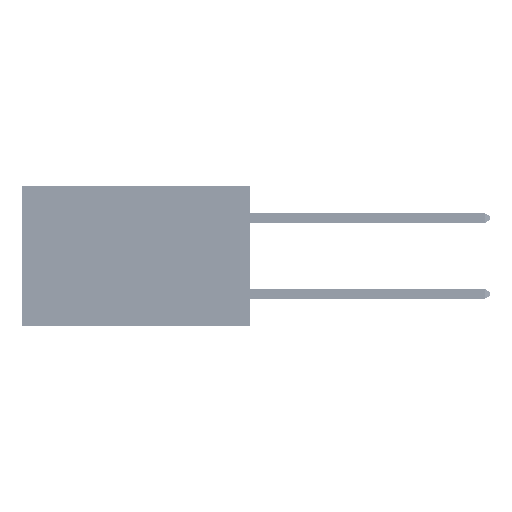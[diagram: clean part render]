
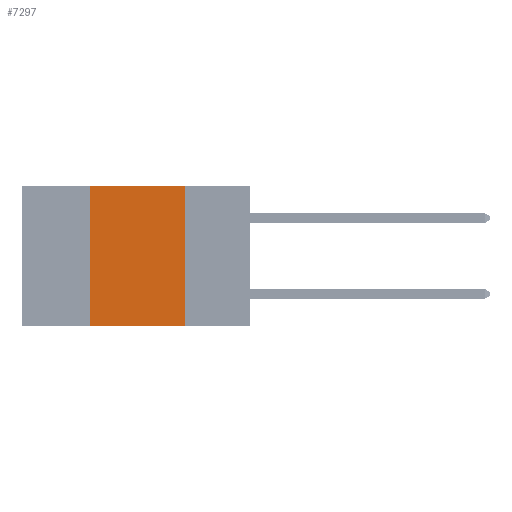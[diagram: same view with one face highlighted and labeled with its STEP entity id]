
A CAD part, left-side view. The second image highlights one B-rep face of the part: STEP entity #7297.
In plain terms, the highlighted planar face has unit normal (-1, 0, 0).
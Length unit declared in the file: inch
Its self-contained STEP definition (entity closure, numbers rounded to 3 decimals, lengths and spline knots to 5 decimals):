
#2633 = VERTEX_POINT ( 'NONE', #10321 ) ;
#2894 = ORIENTED_EDGE ( 'NONE', *, *, #41545, .F. ) ;
#4387 = CARTESIAN_POINT ( 'NONE',  ( 0., 0.17, 0. ) ) ;
#5004 = VECTOR ( 'NONE', #29606, 39.37008 ) ;
#6440 = ORIENTED_EDGE ( 'NONE', *, *, #28216, .T. ) ;
#6649 = CARTESIAN_POINT ( 'NONE',  ( 0., 0.42, 0. ) ) ;
#7297 = ADVANCED_FACE ( 'NONE', ( #26547 ), #14944, .F. ) ;
#7393 = CARTESIAN_POINT ( 'NONE',  ( 0., 0.6, 0. ) ) ;
#8429 = DIRECTION ( 'NONE',  ( 0., 0., -1. ) ) ;
#8774 = LINE ( 'NONE', #33139, #5004 ) ;
#9118 = DIRECTION ( 'NONE',  ( 0., 0., -1. ) ) ;
#10321 = CARTESIAN_POINT ( 'NONE',  ( 0., 0.17, -0.37 ) ) ;
#12246 = CARTESIAN_POINT ( 'NONE',  ( 0., 0.6, 0. ) ) ;
#13129 = VERTEX_POINT ( 'NONE', #13296 ) ;
#13296 = CARTESIAN_POINT ( 'NONE',  ( 0., 0.42, -0.37 ) ) ;
#14944 = PLANE ( 'NONE',  #26729 ) ;
#20258 = ORIENTED_EDGE ( 'NONE', *, *, #29442, .F. ) ;
#24461 = DIRECTION ( 'NONE',  ( 0., -1., 0. ) ) ;
#26202 = LINE ( 'NONE', #36017, #29356 ) ;
#26547 = FACE_OUTER_BOUND ( 'NONE', #36222, .T. ) ;
#26729 = AXIS2_PLACEMENT_3D ( 'NONE', #7393, #36523, #9118 ) ;
#28216 = EDGE_CURVE ( 'NONE', #13129, #2633, #8774, .T. ) ;
#29218 = LINE ( 'NONE', #12246, #41192 ) ;
#29356 = VECTOR ( 'NONE', #31941, 39.37008 ) ;
#29442 = EDGE_CURVE ( 'NONE', #32370, #2633, #43168, .T. ) ;
#29606 = DIRECTION ( 'NONE',  ( 0., -1., 0. ) ) ;
#29958 = ORIENTED_EDGE ( 'NONE', *, *, #34683, .F. ) ;
#31941 = DIRECTION ( 'NONE',  ( 0., 0., 1. ) ) ;
#32370 = VERTEX_POINT ( 'NONE', #51490 ) ;
#33139 = CARTESIAN_POINT ( 'NONE',  ( 0., 0.6, -0.37 ) ) ;
#34683 = EDGE_CURVE ( 'NONE', #38655, #32370, #29218, .T. ) ;
#36017 = CARTESIAN_POINT ( 'NONE',  ( 0., 0.42, 0. ) ) ;
#36222 = EDGE_LOOP ( 'NONE', ( #20258, #29958, #2894, #6440 ) ) ;
#36523 = DIRECTION ( 'NONE',  ( 1., 0., 0. ) ) ;
#38655 = VERTEX_POINT ( 'NONE', #6649 ) ;
#41192 = VECTOR ( 'NONE', #24461, 39.37008 ) ;
#41545 = EDGE_CURVE ( 'NONE', #13129, #38655, #26202, .T. ) ;
#43168 = LINE ( 'NONE', #4387, #46278 ) ;
#46278 = VECTOR ( 'NONE', #8429, 39.37008 ) ;
#51490 = CARTESIAN_POINT ( 'NONE',  ( 0., 0.17, 0. ) ) ;
